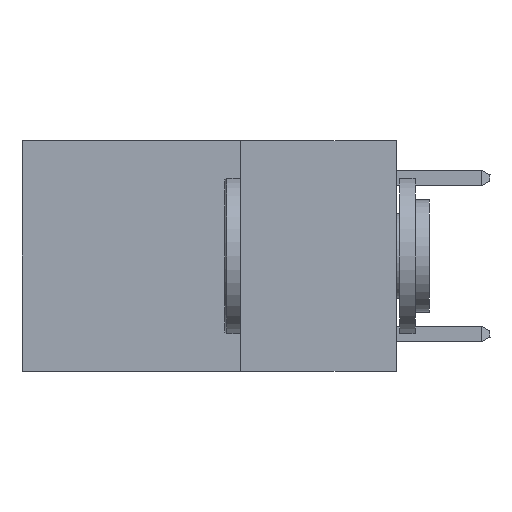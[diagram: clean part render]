
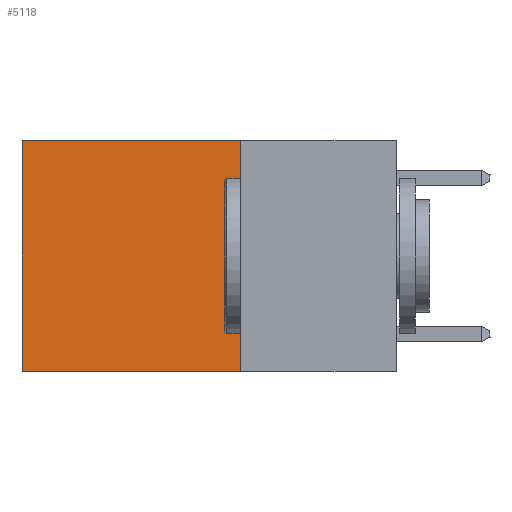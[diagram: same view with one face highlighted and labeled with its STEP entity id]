
A CAD part, left-side view. The second image highlights one B-rep face of the part: STEP entity #5118.
In plain terms, the highlighted planar face has unit normal (-1, 0, 0).
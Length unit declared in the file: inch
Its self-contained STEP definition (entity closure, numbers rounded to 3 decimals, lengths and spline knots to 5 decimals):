
#1088 = CARTESIAN_POINT ( 'NONE',  ( 0.2625, 0.25, 0. ) ) ;
#1969 = CARTESIAN_POINT ( 'NONE',  ( 0.2625, 0.25, -0.37 ) ) ;
#3527 = EDGE_CURVE ( 'NONE', #20451, #14372, #18142, .T. ) ;
#3987 = ORIENTED_EDGE ( 'NONE', *, *, #19021, .T. ) ;
#5118 = ADVANCED_FACE ( 'NONE', ( #16430 ), #12918, .F. ) ;
#5329 = DIRECTION ( 'NONE',  ( 0., 0., -1. ) ) ;
#5690 = DIRECTION ( 'NONE',  ( 1., 0., 0. ) ) ;
#6623 = EDGE_CURVE ( 'NONE', #14372, #21063, #18872, .T. ) ;
#9389 = ORIENTED_EDGE ( 'NONE', *, *, #3527, .F. ) ;
#9547 = AXIS2_PLACEMENT_3D ( 'NONE', #14499, #5690, #5329 ) ;
#10260 = LINE ( 'NONE', #21125, #20809 ) ;
#12918 = PLANE ( 'NONE',  #9547 ) ;
#12939 = DIRECTION ( 'NONE',  ( 0., 0., -1. ) ) ;
#14372 = VERTEX_POINT ( 'NONE', #23365 ) ;
#14499 = CARTESIAN_POINT ( 'NONE',  ( 0.2625, 0.25, 0. ) ) ;
#14936 = VERTEX_POINT ( 'NONE', #16677 ) ;
#15140 = ORIENTED_EDGE ( 'NONE', *, *, #6623, .F. ) ;
#15208 = EDGE_LOOP ( 'NONE', ( #19814, #15140, #9389, #3987 ) ) ;
#16336 = LINE ( 'NONE', #16700, #21612 ) ;
#16430 = FACE_OUTER_BOUND ( 'NONE', #15208, .T. ) ;
#16677 = CARTESIAN_POINT ( 'NONE',  ( 0.2625, 0.6, 0. ) ) ;
#16700 = CARTESIAN_POINT ( 'NONE',  ( 0.2625, 0.6, 0. ) ) ;
#18142 = LINE ( 'NONE', #23821, #23466 ) ;
#18872 = LINE ( 'NONE', #1969, #23640 ) ;
#19021 = EDGE_CURVE ( 'NONE', #20451, #14936, #10260, .T. ) ;
#19814 = ORIENTED_EDGE ( 'NONE', *, *, #20314, .T. ) ;
#20314 = EDGE_CURVE ( 'NONE', #14936, #21063, #16336, .T. ) ;
#20451 = VERTEX_POINT ( 'NONE', #1088 ) ;
#20809 = VECTOR ( 'NONE', #22940, 39.37008 ) ;
#21063 = VERTEX_POINT ( 'NONE', #21803 ) ;
#21125 = CARTESIAN_POINT ( 'NONE',  ( 0.2625, 0.25, 0. ) ) ;
#21612 = VECTOR ( 'NONE', #23710, 39.37008 ) ;
#21803 = CARTESIAN_POINT ( 'NONE',  ( 0.2625, 0.6, -0.37 ) ) ;
#22254 = DIRECTION ( 'NONE',  ( 0., 1., 0. ) ) ;
#22940 = DIRECTION ( 'NONE',  ( 0., 1., 0. ) ) ;
#23365 = CARTESIAN_POINT ( 'NONE',  ( 0.2625, 0.25, -0.37 ) ) ;
#23466 = VECTOR ( 'NONE', #12939, 39.37008 ) ;
#23640 = VECTOR ( 'NONE', #22254, 39.37008 ) ;
#23710 = DIRECTION ( 'NONE',  ( 0., 0., -1. ) ) ;
#23821 = CARTESIAN_POINT ( 'NONE',  ( 0.2625, 0.25, 0. ) ) ;
